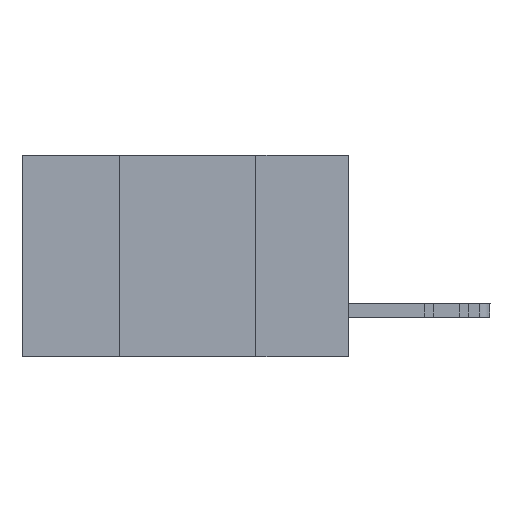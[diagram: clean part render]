
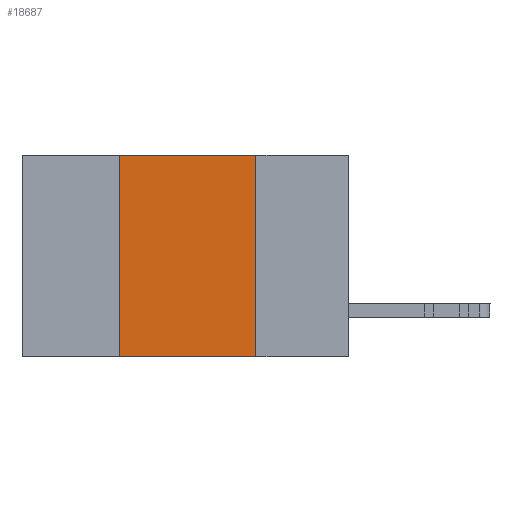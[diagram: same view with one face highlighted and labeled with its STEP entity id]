
A CAD part, left-side view. The second image highlights one B-rep face of the part: STEP entity #18687.
In plain terms, the highlighted planar face has unit normal (-1, 0, 0).
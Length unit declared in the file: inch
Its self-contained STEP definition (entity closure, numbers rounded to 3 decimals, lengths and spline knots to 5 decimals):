
#641 = ORIENTED_EDGE ( 'NONE', *, *, #5107, .F. ) ;
#1173 = ORIENTED_EDGE ( 'NONE', *, *, #21926, .T. ) ;
#1443 = CARTESIAN_POINT ( 'NONE',  ( 0., 0.6, 0. ) ) ;
#2352 = VECTOR ( 'NONE', #6611, 39.37008 ) ;
#3424 = VERTEX_POINT ( 'NONE', #14690 ) ;
#4590 = CARTESIAN_POINT ( 'NONE',  ( 0., 0.6, -0.37 ) ) ;
#4714 = DIRECTION ( 'NONE',  ( 0., -1., 0. ) ) ;
#5107 = EDGE_CURVE ( 'NONE', #3424, #18973, #21427, .T. ) ;
#5414 = EDGE_LOOP ( 'NONE', ( #19454, #23746, #641, #1173 ) ) ;
#5425 = PLANE ( 'NONE',  #12588 ) ;
#5513 = DIRECTION ( 'NONE',  ( 0., 0., -1. ) ) ;
#6295 = FACE_OUTER_BOUND ( 'NONE', #5414, .T. ) ;
#6611 = DIRECTION ( 'NONE',  ( 0., -1., 0. ) ) ;
#7139 = DIRECTION ( 'NONE',  ( 0., 0., 1. ) ) ;
#7225 = CARTESIAN_POINT ( 'NONE',  ( 0., 0.42, -0.37 ) ) ;
#8172 = VECTOR ( 'NONE', #24794, 39.37008 ) ;
#11046 = CARTESIAN_POINT ( 'NONE',  ( 0., 0.17, -0.37 ) ) ;
#11339 = VERTEX_POINT ( 'NONE', #17046 ) ;
#12588 = AXIS2_PLACEMENT_3D ( 'NONE', #1443, #17559, #5513 ) ;
#12667 = CARTESIAN_POINT ( 'NONE',  ( 0., 0.42, 0. ) ) ;
#13092 = LINE ( 'NONE', #4590, #2352 ) ;
#13499 = LINE ( 'NONE', #11046, #8172 ) ;
#13602 = EDGE_CURVE ( 'NONE', #18417, #11339, #13499, .T. ) ;
#14690 = CARTESIAN_POINT ( 'NONE',  ( 0., 0.42, -0.37 ) ) ;
#14734 = CARTESIAN_POINT ( 'NONE',  ( 0., 0.17, 0. ) ) ;
#16862 = VECTOR ( 'NONE', #7139, 39.37008 ) ;
#17046 = CARTESIAN_POINT ( 'NONE',  ( 0., 0.17, -0.37 ) ) ;
#17559 = DIRECTION ( 'NONE',  ( 1., 0., 0. ) ) ;
#18417 = VERTEX_POINT ( 'NONE', #14734 ) ;
#18687 = ADVANCED_FACE ( 'NONE', ( #6295 ), #5425, .F. ) ;
#18779 = CARTESIAN_POINT ( 'NONE',  ( 0., 0.6, 0. ) ) ;
#18973 = VERTEX_POINT ( 'NONE', #12667 ) ;
#19454 = ORIENTED_EDGE ( 'NONE', *, *, #13602, .F. ) ;
#20284 = LINE ( 'NONE', #18779, #24712 ) ;
#20858 = EDGE_CURVE ( 'NONE', #18973, #18417, #20284, .T. ) ;
#21427 = LINE ( 'NONE', #7225, #16862 ) ;
#21926 = EDGE_CURVE ( 'NONE', #3424, #11339, #13092, .T. ) ;
#23746 = ORIENTED_EDGE ( 'NONE', *, *, #20858, .F. ) ;
#24712 = VECTOR ( 'NONE', #4714, 39.37008 ) ;
#24794 = DIRECTION ( 'NONE',  ( 0., 0., -1. ) ) ;
